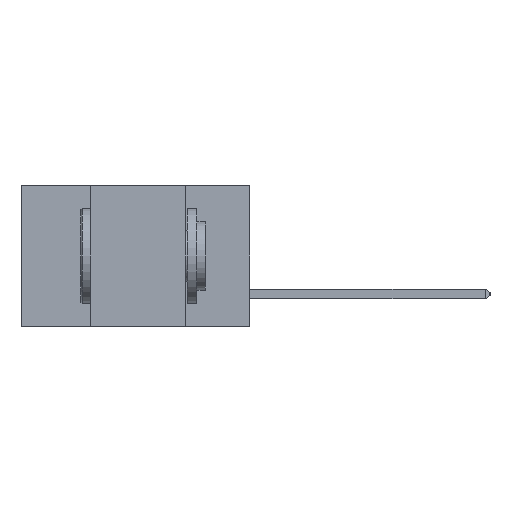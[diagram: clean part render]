
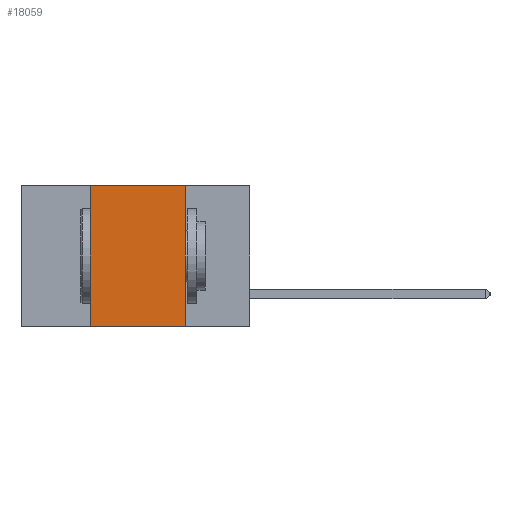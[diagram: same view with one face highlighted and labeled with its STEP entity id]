
A CAD part, left-side view. The second image highlights one B-rep face of the part: STEP entity #18059.
In plain terms, the highlighted planar face has unit normal (-1, 0, 0).
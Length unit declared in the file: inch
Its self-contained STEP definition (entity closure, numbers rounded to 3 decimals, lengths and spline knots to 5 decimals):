
#457 = CARTESIAN_POINT ( 'NONE',  ( 0., 0.17, 0. ) ) ;
#812 = VERTEX_POINT ( 'NONE', #457 ) ;
#2152 = LINE ( 'NONE', #13220, #17109 ) ;
#2345 = DIRECTION ( 'NONE',  ( 0., 0., 1. ) ) ;
#2363 = DIRECTION ( 'NONE',  ( 1., 0., 0. ) ) ;
#4364 = CARTESIAN_POINT ( 'NONE',  ( 0., 0.42, -0.37 ) ) ;
#4755 = VERTEX_POINT ( 'NONE', #15380 ) ;
#5457 = CARTESIAN_POINT ( 'NONE',  ( 0., 0.42, 0. ) ) ;
#5712 = AXIS2_PLACEMENT_3D ( 'NONE', #11143, #2363, #12580 ) ;
#6065 = DIRECTION ( 'NONE',  ( 0., -1., 0. ) ) ;
#6243 = VECTOR ( 'NONE', #18464, 39.37008 ) ;
#6473 = LINE ( 'NONE', #15743, #16971 ) ;
#7179 = LINE ( 'NONE', #9999, #6243 ) ;
#7487 = EDGE_CURVE ( 'NONE', #812, #4755, #7179, .T. ) ;
#9707 = PLANE ( 'NONE',  #5712 ) ;
#9999 = CARTESIAN_POINT ( 'NONE',  ( 0., 0.17, 0. ) ) ;
#10327 = EDGE_CURVE ( 'NONE', #16308, #812, #2152, .T. ) ;
#11143 = CARTESIAN_POINT ( 'NONE',  ( 0., 0.6, 0. ) ) ;
#11260 = ORIENTED_EDGE ( 'NONE', *, *, #14431, .T. ) ;
#11893 = ORIENTED_EDGE ( 'NONE', *, *, #7487, .F. ) ;
#12431 = EDGE_LOOP ( 'NONE', ( #11893, #16074, #12497, #11260 ) ) ;
#12497 = ORIENTED_EDGE ( 'NONE', *, *, #12533, .F. ) ;
#12533 = EDGE_CURVE ( 'NONE', #17674, #16308, #17441, .T. ) ;
#12580 = DIRECTION ( 'NONE',  ( 0., 0., -1. ) ) ;
#13220 = CARTESIAN_POINT ( 'NONE',  ( 0., 0.6, 0. ) ) ;
#14362 = DIRECTION ( 'NONE',  ( 0., -1., 0. ) ) ;
#14431 = EDGE_CURVE ( 'NONE', #17674, #4755, #6473, .T. ) ;
#15380 = CARTESIAN_POINT ( 'NONE',  ( 0., 0.17, -0.37 ) ) ;
#15743 = CARTESIAN_POINT ( 'NONE',  ( 0., 0.6, -0.37 ) ) ;
#16074 = ORIENTED_EDGE ( 'NONE', *, *, #10327, .F. ) ;
#16308 = VERTEX_POINT ( 'NONE', #5457 ) ;
#16586 = VECTOR ( 'NONE', #2345, 39.37008 ) ;
#16729 = FACE_OUTER_BOUND ( 'NONE', #12431, .T. ) ;
#16971 = VECTOR ( 'NONE', #14362, 39.37008 ) ;
#17109 = VECTOR ( 'NONE', #6065, 39.37008 ) ;
#17441 = LINE ( 'NONE', #18152, #16586 ) ;
#17674 = VERTEX_POINT ( 'NONE', #4364 ) ;
#18059 = ADVANCED_FACE ( 'NONE', ( #16729 ), #9707, .F. ) ;
#18152 = CARTESIAN_POINT ( 'NONE',  ( 0., 0.42, 0. ) ) ;
#18464 = DIRECTION ( 'NONE',  ( 0., 0., -1. ) ) ;
